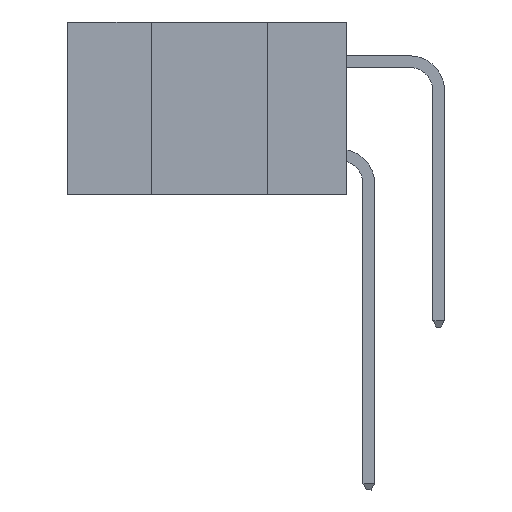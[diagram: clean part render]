
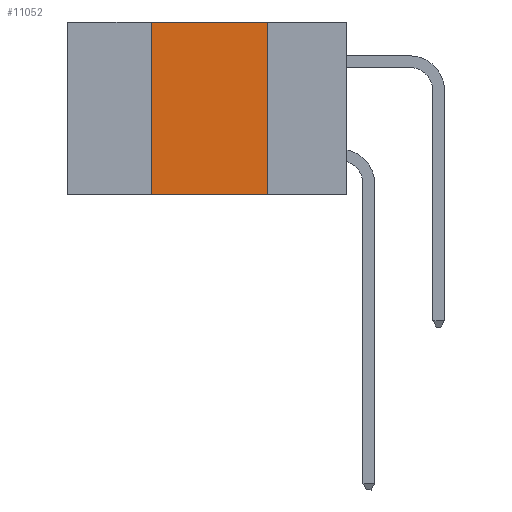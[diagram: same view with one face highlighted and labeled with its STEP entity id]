
A CAD part, left-side view. The second image highlights one B-rep face of the part: STEP entity #11052.
In plain terms, the highlighted planar face has unit normal (-1, 0, 0).
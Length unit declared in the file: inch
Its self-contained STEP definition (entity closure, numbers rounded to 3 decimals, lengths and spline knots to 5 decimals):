
#2369 = LINE ( 'NONE', #11109, #23320 ) ;
#4383 = ORIENTED_EDGE ( 'NONE', *, *, #7591, .T. ) ;
#5054 = DIRECTION ( 'NONE',  ( 0., -1., 0. ) ) ;
#5467 = VERTEX_POINT ( 'NONE', #37658 ) ;
#5864 = LINE ( 'NONE', #34447, #11769 ) ;
#7591 = EDGE_CURVE ( 'NONE', #5467, #14169, #2369, .T. ) ;
#8989 = CARTESIAN_POINT ( 'NONE',  ( 0., 0.17, 0. ) ) ;
#9856 = LINE ( 'NONE', #15736, #33993 ) ;
#11052 = ADVANCED_FACE ( 'NONE', ( #20370 ), #33137, .F. ) ;
#11109 = CARTESIAN_POINT ( 'NONE',  ( 0., 0.6, -0.37 ) ) ;
#11769 = VECTOR ( 'NONE', #18377, 39.37008 ) ;
#14169 = VERTEX_POINT ( 'NONE', #25080 ) ;
#14446 = DIRECTION ( 'NONE',  ( 0., -1., 0. ) ) ;
#14906 = EDGE_CURVE ( 'NONE', #28841, #41850, #9856, .T. ) ;
#15736 = CARTESIAN_POINT ( 'NONE',  ( 0., 0.6, 0. ) ) ;
#15843 = DIRECTION ( 'NONE',  ( 0., 0., 1. ) ) ;
#17681 = EDGE_LOOP ( 'NONE', ( #39759, #27277, #35534, #4383 ) ) ;
#18377 = DIRECTION ( 'NONE',  ( 0., 0., -1. ) ) ;
#20370 = FACE_OUTER_BOUND ( 'NONE', #17681, .T. ) ;
#22492 = DIRECTION ( 'NONE',  ( 1., 0., 0. ) ) ;
#23320 = VECTOR ( 'NONE', #14446, 39.37008 ) ;
#24491 = EDGE_CURVE ( 'NONE', #5467, #28841, #31615, .T. ) ;
#25080 = CARTESIAN_POINT ( 'NONE',  ( 0., 0.17, -0.37 ) ) ;
#25353 = CARTESIAN_POINT ( 'NONE',  ( 0., 0.42, 0. ) ) ;
#27277 = ORIENTED_EDGE ( 'NONE', *, *, #14906, .F. ) ;
#28841 = VERTEX_POINT ( 'NONE', #25353 ) ;
#31615 = LINE ( 'NONE', #36364, #35361 ) ;
#33137 = PLANE ( 'NONE',  #35758 ) ;
#33298 = DIRECTION ( 'NONE',  ( 0., 0., -1. ) ) ;
#33993 = VECTOR ( 'NONE', #5054, 39.37008 ) ;
#34379 = EDGE_CURVE ( 'NONE', #41850, #14169, #5864, .T. ) ;
#34447 = CARTESIAN_POINT ( 'NONE',  ( 0., 0.17, 0. ) ) ;
#35361 = VECTOR ( 'NONE', #15843, 39.37008 ) ;
#35534 = ORIENTED_EDGE ( 'NONE', *, *, #24491, .F. ) ;
#35758 = AXIS2_PLACEMENT_3D ( 'NONE', #39755, #22492, #33298 ) ;
#36364 = CARTESIAN_POINT ( 'NONE',  ( 0., 0.42, 0. ) ) ;
#37658 = CARTESIAN_POINT ( 'NONE',  ( 0., 0.42, -0.37 ) ) ;
#39755 = CARTESIAN_POINT ( 'NONE',  ( 0., 0.6, 0. ) ) ;
#39759 = ORIENTED_EDGE ( 'NONE', *, *, #34379, .F. ) ;
#41850 = VERTEX_POINT ( 'NONE', #8989 ) ;
